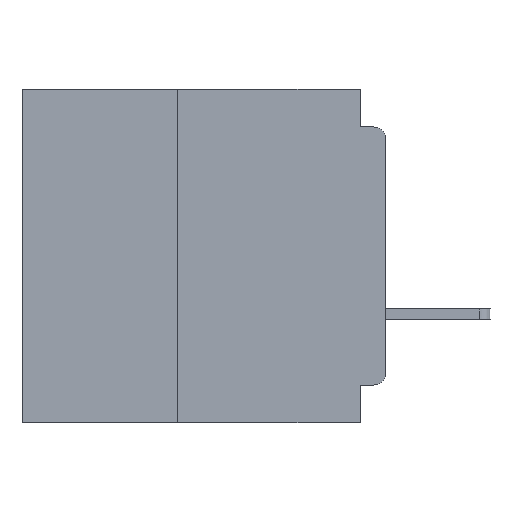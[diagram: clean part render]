
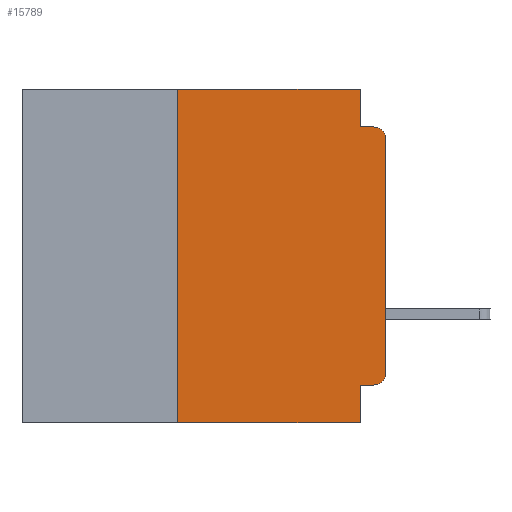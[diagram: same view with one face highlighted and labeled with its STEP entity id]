
A CAD part, left-side view. The second image highlights one B-rep face of the part: STEP entity #15789.
In plain terms, the highlighted planar face has unit normal (-1, 0, 0).
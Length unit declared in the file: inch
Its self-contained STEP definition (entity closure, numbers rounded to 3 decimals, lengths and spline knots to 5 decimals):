
#408 = DIRECTION ( 'NONE',  ( 0., 0., 1. ) ) ;
#1376 = AXIS2_PLACEMENT_3D ( 'NONE', #36957, #5657, #42133 ) ;
#1732 = VERTEX_POINT ( 'NONE', #56387 ) ;
#2009 = ORIENTED_EDGE ( 'NONE', *, *, #21546, .F. ) ;
#4605 = VECTOR ( 'NONE', #47965, 39.37008 ) ;
#5657 = DIRECTION ( 'NONE',  ( -1., 0., 0. ) ) ;
#5710 = CARTESIAN_POINT ( 'NONE',  ( 0., 0.25, -0.4 ) ) ;
#6450 = EDGE_CURVE ( 'NONE', #22764, #27157, #54761, .T. ) ;
#6704 = EDGE_CURVE ( 'NONE', #7739, #60466, #9828, .T. ) ;
#6908 = FACE_OUTER_BOUND ( 'NONE', #50315, .T. ) ;
#7739 = VERTEX_POINT ( 'NONE', #52530 ) ;
#9828 = CIRCLE ( 'NONE', #50242, 0.015 ) ;
#10246 = VERTEX_POINT ( 'NONE', #54645 ) ;
#11448 = VECTOR ( 'NONE', #11483, 39.37008 ) ;
#11483 = DIRECTION ( 'NONE',  ( 0., -1., 0. ) ) ;
#11595 = CARTESIAN_POINT ( 'NONE',  ( 0., 0.031, -0.4 ) ) ;
#12591 = CARTESIAN_POINT ( 'NONE',  ( 0., 0.031, -0.4 ) ) ;
#13244 = EDGE_CURVE ( 'NONE', #27157, #7739, #47234, .T. ) ;
#13915 = EDGE_CURVE ( 'NONE', #10246, #1732, #43076, .T. ) ;
#13951 = ORIENTED_EDGE ( 'NONE', *, *, #32521, .F. ) ;
#13959 = CARTESIAN_POINT ( 'NONE',  ( 0., 0.031, 0. ) ) ;
#14281 = LINE ( 'NONE', #60974, #40371 ) ;
#14848 = CARTESIAN_POINT ( 'NONE',  ( 0., 0., -0.34 ) ) ;
#15789 = ADVANCED_FACE ( 'NONE', ( #6908 ), #61338, .F. ) ;
#19962 = AXIS2_PLACEMENT_3D ( 'NONE', #25181, #30408, #66554 ) ;
#20161 = VERTEX_POINT ( 'NONE', #12591 ) ;
#21546 = EDGE_CURVE ( 'NONE', #22764, #48345, #14281, .T. ) ;
#22764 = VERTEX_POINT ( 'NONE', #23684 ) ;
#23475 = DIRECTION ( 'NONE',  ( -1., 0., 0. ) ) ;
#23684 = CARTESIAN_POINT ( 'NONE',  ( 0., 0.015, -0.355 ) ) ;
#23976 = VECTOR ( 'NONE', #408, 39.37008 ) ;
#24028 = ORIENTED_EDGE ( 'NONE', *, *, #46925, .F. ) ;
#24794 = DIRECTION ( 'NONE',  ( 0., 1., 0. ) ) ;
#25181 = CARTESIAN_POINT ( 'NONE',  ( 0., 0.437, 0. ) ) ;
#26280 = ORIENTED_EDGE ( 'NONE', *, *, #45712, .F. ) ;
#26608 = CARTESIAN_POINT ( 'NONE',  ( 0., 0., -0.045 ) ) ;
#27157 = VERTEX_POINT ( 'NONE', #14848 ) ;
#28213 = LINE ( 'NONE', #55723, #40399 ) ;
#30408 = DIRECTION ( 'NONE',  ( 1., 0., 0. ) ) ;
#30592 = VERTEX_POINT ( 'NONE', #32218 ) ;
#32166 = CARTESIAN_POINT ( 'NONE',  ( 0., 0.015, -0.045 ) ) ;
#32218 = CARTESIAN_POINT ( 'NONE',  ( 0., 0.25, 0. ) ) ;
#32521 = EDGE_CURVE ( 'NONE', #41061, #30592, #54768, .T. ) ;
#34249 = EDGE_CURVE ( 'NONE', #41061, #20161, #39186, .T. ) ;
#36957 = CARTESIAN_POINT ( 'NONE',  ( 0., 0.015, -0.34 ) ) ;
#38676 = ORIENTED_EDGE ( 'NONE', *, *, #13915, .F. ) ;
#39186 = LINE ( 'NONE', #42462, #11448 ) ;
#40166 = ORIENTED_EDGE ( 'NONE', *, *, #6450, .T. ) ;
#40371 = VECTOR ( 'NONE', #24794, 39.37008 ) ;
#40399 = VECTOR ( 'NONE', #66135, 39.37008 ) ;
#41061 = VERTEX_POINT ( 'NONE', #46428 ) ;
#41491 = VECTOR ( 'NONE', #52594, 39.37008 ) ;
#42133 = DIRECTION ( 'NONE',  ( 0., 0., -1. ) ) ;
#42462 = CARTESIAN_POINT ( 'NONE',  ( 0., 0.437, -0.4 ) ) ;
#43076 = LINE ( 'NONE', #13959, #55160 ) ;
#43103 = LINE ( 'NONE', #26608, #41491 ) ;
#43883 = DIRECTION ( 'NONE',  ( 0., 0., 1. ) ) ;
#45712 = EDGE_CURVE ( 'NONE', #1732, #60466, #43103, .T. ) ;
#46428 = CARTESIAN_POINT ( 'NONE',  ( 0., 0.25, -0.4 ) ) ;
#46762 = ORIENTED_EDGE ( 'NONE', *, *, #13244, .T. ) ;
#46925 = EDGE_CURVE ( 'NONE', #48345, #20161, #59856, .T. ) ;
#47088 = ORIENTED_EDGE ( 'NONE', *, *, #6704, .T. ) ;
#47234 = LINE ( 'NONE', #49039, #59310 ) ;
#47965 = DIRECTION ( 'NONE',  ( 0., 0., -1. ) ) ;
#48345 = VERTEX_POINT ( 'NONE', #56863 ) ;
#49039 = CARTESIAN_POINT ( 'NONE',  ( 0., 0., 0. ) ) ;
#50242 = AXIS2_PLACEMENT_3D ( 'NONE', #54474, #23475, #59671 ) ;
#50315 = EDGE_LOOP ( 'NONE', ( #46762, #47088, #26280, #38676, #60368, #13951, #60035, #24028, #2009, #40166 ) ) ;
#52530 = CARTESIAN_POINT ( 'NONE',  ( 0., 0., -0.06 ) ) ;
#52594 = DIRECTION ( 'NONE',  ( 0., -1., 0. ) ) ;
#52843 = EDGE_CURVE ( 'NONE', #30592, #10246, #28213, .T. ) ;
#54474 = CARTESIAN_POINT ( 'NONE',  ( 0., 0.015, -0.06 ) ) ;
#54645 = CARTESIAN_POINT ( 'NONE',  ( 0., 0.031, 0. ) ) ;
#54761 = CIRCLE ( 'NONE', #1376, 0.015 ) ;
#54768 = LINE ( 'NONE', #5710, #23976 ) ;
#55160 = VECTOR ( 'NONE', #60440, 39.37008 ) ;
#55723 = CARTESIAN_POINT ( 'NONE',  ( 0., 0.437, 0. ) ) ;
#56387 = CARTESIAN_POINT ( 'NONE',  ( 0., 0.031, -0.045 ) ) ;
#56863 = CARTESIAN_POINT ( 'NONE',  ( 0., 0.031, -0.355 ) ) ;
#59310 = VECTOR ( 'NONE', #43883, 39.37008 ) ;
#59671 = DIRECTION ( 'NONE',  ( 0., 0., -1. ) ) ;
#59856 = LINE ( 'NONE', #11595, #4605 ) ;
#60035 = ORIENTED_EDGE ( 'NONE', *, *, #34249, .T. ) ;
#60368 = ORIENTED_EDGE ( 'NONE', *, *, #52843, .F. ) ;
#60440 = DIRECTION ( 'NONE',  ( 0., 0., -1. ) ) ;
#60466 = VERTEX_POINT ( 'NONE', #32166 ) ;
#60974 = CARTESIAN_POINT ( 'NONE',  ( 0., 0., -0.355 ) ) ;
#61338 = PLANE ( 'NONE',  #19962 ) ;
#66135 = DIRECTION ( 'NONE',  ( 0., -1., 0. ) ) ;
#66554 = DIRECTION ( 'NONE',  ( 0., 0., -1. ) ) ;
